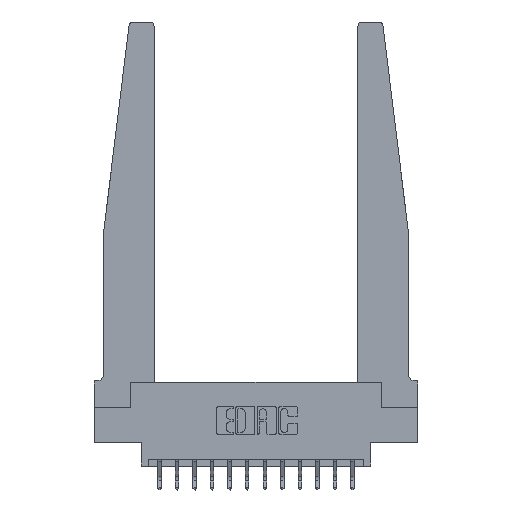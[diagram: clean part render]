
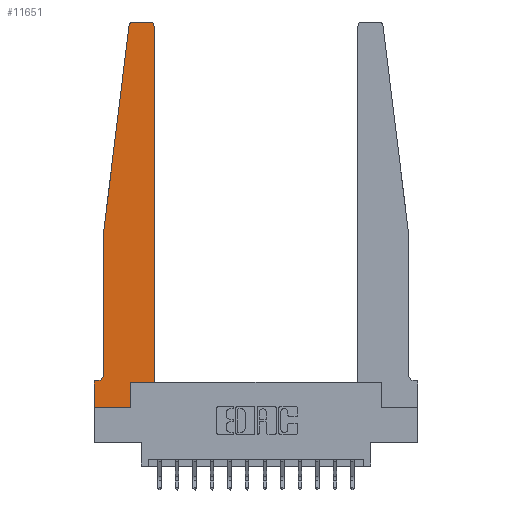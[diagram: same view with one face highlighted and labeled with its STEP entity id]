
A CAD part, top view. The second image highlights one B-rep face of the part: STEP entity #11651.
In plain terms, the highlighted planar face has unit normal (0, 0, 1).
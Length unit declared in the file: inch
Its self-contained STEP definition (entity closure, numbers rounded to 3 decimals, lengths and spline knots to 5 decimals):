
#5 = CARTESIAN_POINT ( 'NONE',  ( 0.425, 0.18, 0.37 ) ) ;
#169 = CARTESIAN_POINT ( 'NONE',  ( 0.395, 2.72, 0.37 ) ) ;
#171 = AXIS2_PLACEMENT_3D ( 'NONE', #15221, #5813, #5907 ) ;
#172 = DIRECTION ( 'NONE',  ( 0., 1., 0. ) ) ;
#233 = EDGE_CURVE ( 'NONE', #6673, #2907, #15277, .T. ) ;
#254 = CIRCLE ( 'NONE', #2538, 0.05 ) ;
#791 = EDGE_CURVE ( 'NONE', #15963, #12739, #8032, .T. ) ;
#1605 = DIRECTION ( 'NONE',  ( -0.122, -0.992, 0. ) ) ;
#1672 = DIRECTION ( 'NONE',  ( 0., 0., 1. ) ) ;
#1712 = ORIENTED_EDGE ( 'NONE', *, *, #791, .T. ) ;
#1920 = AXIS2_PLACEMENT_3D ( 'NONE', #2966, #1672, #4070 ) ;
#2057 = VERTEX_POINT ( 'NONE', #10637 ) ;
#2065 = CARTESIAN_POINT ( 'NONE',  ( 0.395, 2.75, 0.37 ) ) ;
#2105 = EDGE_CURVE ( 'NONE', #12739, #13685, #9333, .T. ) ;
#2258 = ORIENTED_EDGE ( 'NONE', *, *, #2105, .T. ) ;
#2538 = AXIS2_PLACEMENT_3D ( 'NONE', #4598, #9656, #16534 ) ;
#2759 = EDGE_CURVE ( 'NONE', #9383, #8764, #5407, .T. ) ;
#2790 = LINE ( 'NONE', #5448, #7035 ) ;
#2907 = VERTEX_POINT ( 'NONE', #6382 ) ;
#2966 = CARTESIAN_POINT ( 'NONE',  ( 0., 0.1875, 0.37 ) ) ;
#2975 = VERTEX_POINT ( 'NONE', #13485 ) ;
#3375 = AXIS2_PLACEMENT_3D ( 'NONE', #169, #16505, #5787 ) ;
#3475 = CARTESIAN_POINT ( 'NONE',  ( 0., 0., 0.37 ) ) ;
#4025 = DIRECTION ( 'NONE',  ( 0., 1., 0. ) ) ;
#4070 = DIRECTION ( 'NONE',  ( 1., 0., 0. ) ) ;
#4132 = DIRECTION ( 'NONE',  ( -1., 0., 0. ) ) ;
#4451 = CARTESIAN_POINT ( 'NONE',  ( 0.065, 0.2375, 0.37 ) ) ;
#4598 = CARTESIAN_POINT ( 'NONE',  ( 0.015, 0.2375, 0.37 ) ) ;
#4622 = VECTOR ( 'NONE', #8806, 39.37008 ) ;
#4652 = ORIENTED_EDGE ( 'NONE', *, *, #7791, .T. ) ;
#5330 = VECTOR ( 'NONE', #15785, 39.37008 ) ;
#5407 = LINE ( 'NONE', #11015, #9845 ) ;
#5448 = CARTESIAN_POINT ( 'NONE',  ( 0.25, 2.75, 0.37 ) ) ;
#5533 = VERTEX_POINT ( 'NONE', #2065 ) ;
#5541 = EDGE_CURVE ( 'NONE', #8764, #12891, #13069, .T. ) ;
#5787 = DIRECTION ( 'NONE',  ( 1., 0., 0. ) ) ;
#5813 = DIRECTION ( 'NONE',  ( 0., 0., 1. ) ) ;
#5907 = DIRECTION ( 'NONE',  ( 1., 0., 0. ) ) ;
#6318 = ORIENTED_EDGE ( 'NONE', *, *, #8633, .T. ) ;
#6382 = CARTESIAN_POINT ( 'NONE',  ( 0.425, 0.18, 0.37 ) ) ;
#6673 = VERTEX_POINT ( 'NONE', #10140 ) ;
#7035 = VECTOR ( 'NONE', #4132, 39.37008 ) ;
#7129 = DIRECTION ( 'NONE',  ( 1., 0., 0. ) ) ;
#7206 = EDGE_CURVE ( 'NONE', #12891, #2975, #14022, .T. ) ;
#7207 = ORIENTED_EDGE ( 'NONE', *, *, #7206, .T. ) ;
#7772 = CARTESIAN_POINT ( 'NONE',  ( 0., 0., 0.37 ) ) ;
#7791 = EDGE_CURVE ( 'NONE', #2907, #10146, #12185, .T. ) ;
#8025 = CARTESIAN_POINT ( 'NONE',  ( 0.065, 1.25, 0.37 ) ) ;
#8032 = LINE ( 'NONE', #14990, #14451 ) ;
#8633 = EDGE_CURVE ( 'NONE', #10146, #5533, #12062, .T. ) ;
#8764 = VERTEX_POINT ( 'NONE', #9985 ) ;
#8804 = VECTOR ( 'NONE', #4025, 39.37008 ) ;
#8806 = DIRECTION ( 'NONE',  ( 1., 0., 0. ) ) ;
#9326 = CARTESIAN_POINT ( 'NONE',  ( 0.24675, 2.72367, 0.37 ) ) ;
#9333 = LINE ( 'NONE', #8025, #16590 ) ;
#9383 = VERTEX_POINT ( 'NONE', #12677 ) ;
#9425 = DIRECTION ( 'NONE',  ( -1., 0., 0. ) ) ;
#9656 = DIRECTION ( 'NONE',  ( 0., 0., -1. ) ) ;
#9690 = ORIENTED_EDGE ( 'NONE', *, *, #14029, .T. ) ;
#9704 = CARTESIAN_POINT ( 'NONE',  ( 0.425, 0.18, 0.37 ) ) ;
#9845 = VECTOR ( 'NONE', #9425, 39.37008 ) ;
#9985 = CARTESIAN_POINT ( 'NONE',  ( 0., 0.1875, 0.37 ) ) ;
#9998 = EDGE_CURVE ( 'NONE', #2975, #6673, #15982, .T. ) ;
#10140 = CARTESIAN_POINT ( 'NONE',  ( 0.2605, 0.18, 0.37 ) ) ;
#10146 = VERTEX_POINT ( 'NONE', #12731 ) ;
#10154 = ORIENTED_EDGE ( 'NONE', *, *, #2759, .T. ) ;
#10637 = CARTESIAN_POINT ( 'NONE',  ( 0.27653, 2.75, 0.37 ) ) ;
#11015 = CARTESIAN_POINT ( 'NONE',  ( 0.065, 0.1875, 0.37 ) ) ;
#11651 = ADVANCED_FACE ( 'NONE', ( #12216 ), #16113, .T. ) ;
#12062 = CIRCLE ( 'NONE', #3375, 0.03 ) ;
#12185 = LINE ( 'NONE', #5, #15122 ) ;
#12216 = FACE_OUTER_BOUND ( 'NONE', #17125, .T. ) ;
#12658 = ORIENTED_EDGE ( 'NONE', *, *, #9998, .T. ) ;
#12677 = CARTESIAN_POINT ( 'NONE',  ( 0.015, 0.1875, 0.37 ) ) ;
#12731 = CARTESIAN_POINT ( 'NONE',  ( 0.425, 2.72, 0.37 ) ) ;
#12739 = VERTEX_POINT ( 'NONE', #16541 ) ;
#12891 = VERTEX_POINT ( 'NONE', #16963 ) ;
#13069 = LINE ( 'NONE', #7772, #5330 ) ;
#13156 = EDGE_CURVE ( 'NONE', #5533, #2057, #2790, .T. ) ;
#13485 = CARTESIAN_POINT ( 'NONE',  ( 0.2605, 0., 0.37 ) ) ;
#13541 = VECTOR ( 'NONE', #7129, 39.37008 ) ;
#13685 = VERTEX_POINT ( 'NONE', #4451 ) ;
#14022 = LINE ( 'NONE', #3475, #4622 ) ;
#14029 = EDGE_CURVE ( 'NONE', #2057, #15963, #15412, .T. ) ;
#14175 = ORIENTED_EDGE ( 'NONE', *, *, #16392, .T. ) ;
#14359 = ORIENTED_EDGE ( 'NONE', *, *, #13156, .T. ) ;
#14451 = VECTOR ( 'NONE', #1605, 39.37008 ) ;
#14820 = ORIENTED_EDGE ( 'NONE', *, *, #5541, .T. ) ;
#14870 = ORIENTED_EDGE ( 'NONE', *, *, #233, .T. ) ;
#14990 = CARTESIAN_POINT ( 'NONE',  ( 0.065, 1.25, 0.37 ) ) ;
#15122 = VECTOR ( 'NONE', #172, 39.37008 ) ;
#15221 = CARTESIAN_POINT ( 'NONE',  ( 0.27653, 2.72, 0.37 ) ) ;
#15277 = LINE ( 'NONE', #9704, #13541 ) ;
#15412 = CIRCLE ( 'NONE', #171, 0.03 ) ;
#15785 = DIRECTION ( 'NONE',  ( 0., -1., 0. ) ) ;
#15963 = VERTEX_POINT ( 'NONE', #9326 ) ;
#15982 = LINE ( 'NONE', #16073, #8804 ) ;
#16051 = DIRECTION ( 'NONE',  ( 0., -1., 0. ) ) ;
#16073 = CARTESIAN_POINT ( 'NONE',  ( 0.2605, 0.18, 0.37 ) ) ;
#16113 = PLANE ( 'NONE',  #1920 ) ;
#16392 = EDGE_CURVE ( 'NONE', #13685, #9383, #254, .T. ) ;
#16505 = DIRECTION ( 'NONE',  ( 0., 0., 1. ) ) ;
#16534 = DIRECTION ( 'NONE',  ( -1., 0., 0. ) ) ;
#16541 = CARTESIAN_POINT ( 'NONE',  ( 0.065, 1.25, 0.37 ) ) ;
#16590 = VECTOR ( 'NONE', #16051, 39.37008 ) ;
#16963 = CARTESIAN_POINT ( 'NONE',  ( 0., 0., 0.37 ) ) ;
#17125 = EDGE_LOOP ( 'NONE', ( #14359, #9690, #1712, #2258, #14175, #10154, #14820, #7207, #12658, #14870, #4652, #6318 ) ) ;
